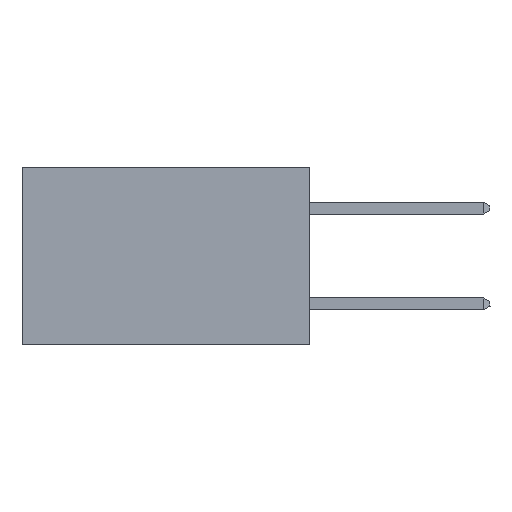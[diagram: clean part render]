
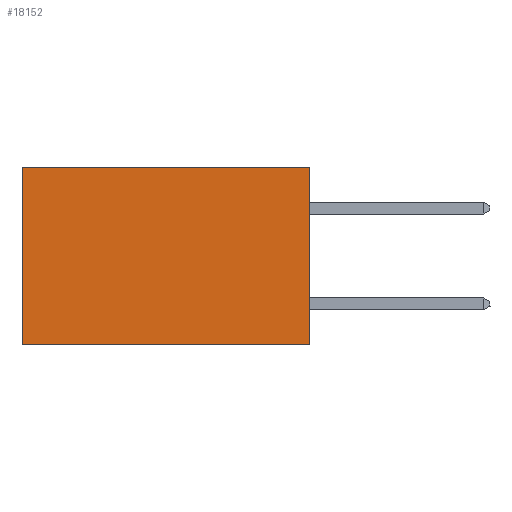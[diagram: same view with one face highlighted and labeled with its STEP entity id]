
A CAD part, left-side view. The second image highlights one B-rep face of the part: STEP entity #18152.
In plain terms, the highlighted planar face has unit normal (-1, 0, 0).
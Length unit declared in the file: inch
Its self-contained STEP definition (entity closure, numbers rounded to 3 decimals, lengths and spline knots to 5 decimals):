
#88 = AXIS2_PLACEMENT_3D ( 'NONE', #22463, #3259, #18064 ) ;
#245 = ORIENTED_EDGE ( 'NONE', *, *, #10165, .F. ) ;
#1744 = EDGE_LOOP ( 'NONE', ( #6859, #245, #15608, #15958 ) ) ;
#3259 = DIRECTION ( 'NONE',  ( 1., 0., 0. ) ) ;
#4985 = DIRECTION ( 'NONE',  ( 0., 0., -1. ) ) ;
#6359 = EDGE_CURVE ( 'NONE', #18426, #18223, #16262, .T. ) ;
#6362 = EDGE_CURVE ( 'NONE', #18426, #17339, #10158, .T. ) ;
#6859 = ORIENTED_EDGE ( 'NONE', *, *, #15865, .T. ) ;
#9614 = CARTESIAN_POINT ( 'NONE',  ( 0.2875, 0., -0.37 ) ) ;
#10158 = LINE ( 'NONE', #21267, #10832 ) ;
#10165 = EDGE_CURVE ( 'NONE', #18223, #13592, #19687, .T. ) ;
#10832 = VECTOR ( 'NONE', #25614, 39.37008 ) ;
#13592 = VERTEX_POINT ( 'NONE', #14727 ) ;
#13662 = PLANE ( 'NONE',  #88 ) ;
#14563 = CARTESIAN_POINT ( 'NONE',  ( 0.2875, 0., 0. ) ) ;
#14727 = CARTESIAN_POINT ( 'NONE',  ( 0.2875, 0.6, -0.37 ) ) ;
#14922 = FACE_OUTER_BOUND ( 'NONE', #1744, .T. ) ;
#15022 = LINE ( 'NONE', #19983, #17338 ) ;
#15608 = ORIENTED_EDGE ( 'NONE', *, *, #6359, .F. ) ;
#15865 = EDGE_CURVE ( 'NONE', #17339, #13592, #15022, .T. ) ;
#15958 = ORIENTED_EDGE ( 'NONE', *, *, #6362, .T. ) ;
#16262 = LINE ( 'NONE', #14563, #25963 ) ;
#16304 = CARTESIAN_POINT ( 'NONE',  ( 0.2875, 0., 0. ) ) ;
#17338 = VECTOR ( 'NONE', #4985, 39.37008 ) ;
#17339 = VERTEX_POINT ( 'NONE', #25471 ) ;
#18064 = DIRECTION ( 'NONE',  ( 0., 0., -1. ) ) ;
#18152 = ADVANCED_FACE ( 'NONE', ( #14922 ), #13662, .F. ) ;
#18223 = VERTEX_POINT ( 'NONE', #9614 ) ;
#18426 = VERTEX_POINT ( 'NONE', #16304 ) ;
#19687 = LINE ( 'NONE', #22657, #22027 ) ;
#19983 = CARTESIAN_POINT ( 'NONE',  ( 0.2875, 0.6, 0. ) ) ;
#21267 = CARTESIAN_POINT ( 'NONE',  ( 0.2875, 0., 0. ) ) ;
#22027 = VECTOR ( 'NONE', #24764, 39.37008 ) ;
#22463 = CARTESIAN_POINT ( 'NONE',  ( 0.2875, 0., 0. ) ) ;
#22657 = CARTESIAN_POINT ( 'NONE',  ( 0.2875, 0., -0.37 ) ) ;
#24764 = DIRECTION ( 'NONE',  ( 0., 1., 0. ) ) ;
#25471 = CARTESIAN_POINT ( 'NONE',  ( 0.2875, 0.6, 0. ) ) ;
#25614 = DIRECTION ( 'NONE',  ( 0., 1., 0. ) ) ;
#25963 = VECTOR ( 'NONE', #27699, 39.37008 ) ;
#27699 = DIRECTION ( 'NONE',  ( 0., 0., -1. ) ) ;
